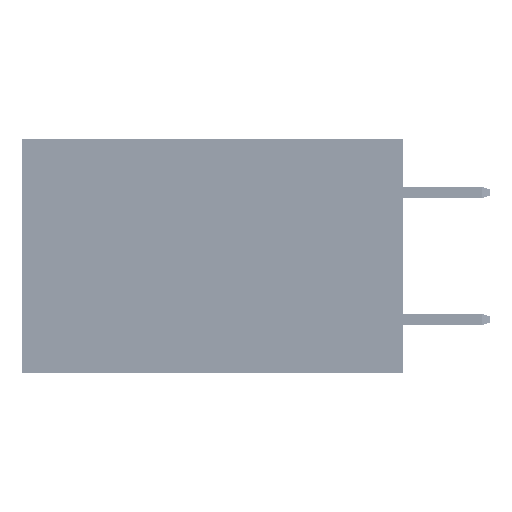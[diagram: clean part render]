
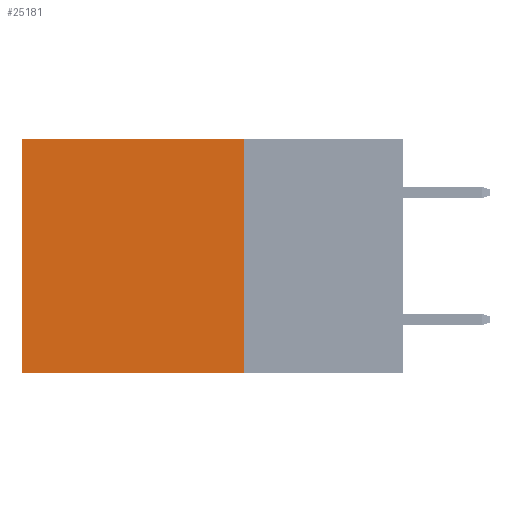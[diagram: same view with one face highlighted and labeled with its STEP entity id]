
A CAD part, left-side view. The second image highlights one B-rep face of the part: STEP entity #25181.
In plain terms, the highlighted planar face has unit normal (-1, 0, 0).
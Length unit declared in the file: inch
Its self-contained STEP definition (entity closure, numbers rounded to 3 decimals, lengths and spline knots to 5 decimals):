
#1405 = AXIS2_PLACEMENT_3D ( 'NONE', #39249, #3279, #26397 ) ;
#1572 = EDGE_CURVE ( 'NONE', #23741, #18698, #24243, .T. ) ;
#3279 = DIRECTION ( 'NONE',  ( 1., 0., 0. ) ) ;
#5076 = VECTOR ( 'NONE', #47676, 39.37008 ) ;
#7758 = LINE ( 'NONE', #31661, #5076 ) ;
#9098 = CARTESIAN_POINT ( 'NONE',  ( 0.2875, 0.6, -0.37 ) ) ;
#9616 = CARTESIAN_POINT ( 'NONE',  ( 0.2875, 0.25, -0.37 ) ) ;
#9728 = EDGE_CURVE ( 'NONE', #40529, #23741, #7758, .T. ) ;
#10436 = EDGE_LOOP ( 'NONE', ( #21343, #13975, #47638, #41530 ) ) ;
#13830 = DIRECTION ( 'NONE',  ( 0., 1., 0. ) ) ;
#13975 = ORIENTED_EDGE ( 'NONE', *, *, #43912, .F. ) ;
#17404 = CARTESIAN_POINT ( 'NONE',  ( 0.2875, 0.6, 0. ) ) ;
#18698 = VERTEX_POINT ( 'NONE', #9098 ) ;
#21343 = ORIENTED_EDGE ( 'NONE', *, *, #1572, .T. ) ;
#21442 = LINE ( 'NONE', #9616, #30811 ) ;
#22512 = DIRECTION ( 'NONE',  ( 0., 0., -1. ) ) ;
#23230 = FACE_OUTER_BOUND ( 'NONE', #10436, .T. ) ;
#23741 = VERTEX_POINT ( 'NONE', #26112 ) ;
#24243 = LINE ( 'NONE', #17404, #29402 ) ;
#25181 = ADVANCED_FACE ( 'NONE', ( #23230 ), #46875, .F. ) ;
#26112 = CARTESIAN_POINT ( 'NONE',  ( 0.2875, 0.6, 0. ) ) ;
#26397 = DIRECTION ( 'NONE',  ( 0., 0., -1. ) ) ;
#29156 = EDGE_CURVE ( 'NONE', #40529, #41825, #30921, .T. ) ;
#29228 = VECTOR ( 'NONE', #22512, 39.37008 ) ;
#29402 = VECTOR ( 'NONE', #44475, 39.37008 ) ;
#30811 = VECTOR ( 'NONE', #13830, 39.37008 ) ;
#30921 = LINE ( 'NONE', #46944, #29228 ) ;
#31661 = CARTESIAN_POINT ( 'NONE',  ( 0.2875, 0.25, 0. ) ) ;
#39249 = CARTESIAN_POINT ( 'NONE',  ( 0.2875, 0.25, 0. ) ) ;
#40529 = VERTEX_POINT ( 'NONE', #45689 ) ;
#41530 = ORIENTED_EDGE ( 'NONE', *, *, #9728, .T. ) ;
#41825 = VERTEX_POINT ( 'NONE', #43859 ) ;
#43859 = CARTESIAN_POINT ( 'NONE',  ( 0.2875, 0.25, -0.37 ) ) ;
#43912 = EDGE_CURVE ( 'NONE', #41825, #18698, #21442, .T. ) ;
#44475 = DIRECTION ( 'NONE',  ( 0., 0., -1. ) ) ;
#45689 = CARTESIAN_POINT ( 'NONE',  ( 0.2875, 0.25, 0. ) ) ;
#46875 = PLANE ( 'NONE',  #1405 ) ;
#46944 = CARTESIAN_POINT ( 'NONE',  ( 0.2875, 0.25, 0. ) ) ;
#47638 = ORIENTED_EDGE ( 'NONE', *, *, #29156, .F. ) ;
#47676 = DIRECTION ( 'NONE',  ( 0., 1., 0. ) ) ;
